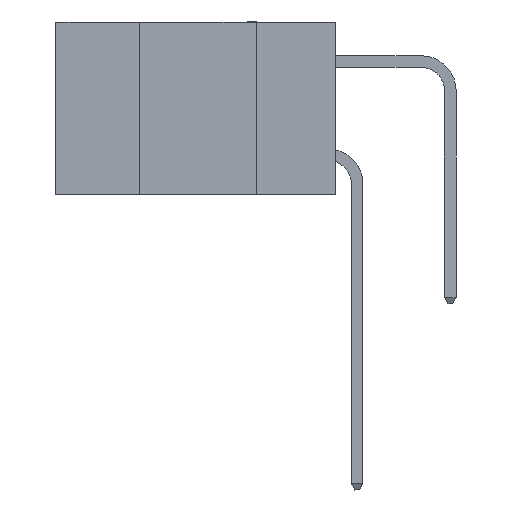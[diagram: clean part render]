
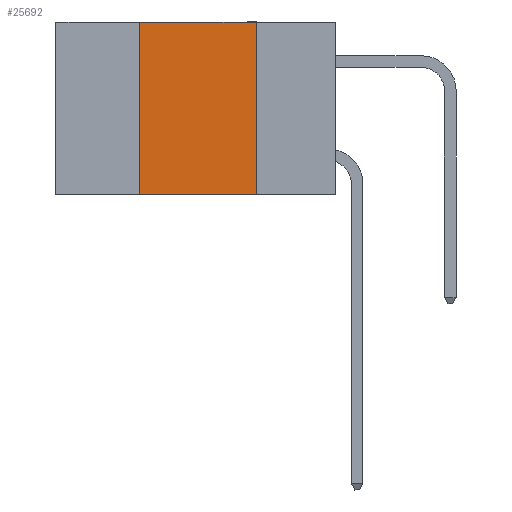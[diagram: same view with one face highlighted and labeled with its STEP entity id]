
A CAD part, left-side view. The second image highlights one B-rep face of the part: STEP entity #25692.
In plain terms, the highlighted planar face has unit normal (-1, 0, 0).
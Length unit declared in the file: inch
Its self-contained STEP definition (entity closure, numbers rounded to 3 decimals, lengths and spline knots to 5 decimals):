
#676 = VERTEX_POINT ( 'NONE', #12379 ) ;
#945 = CARTESIAN_POINT ( 'NONE',  ( 0., 0.17, -0.37 ) ) ;
#1502 = CARTESIAN_POINT ( 'NONE',  ( 0., 0.6, -0.37 ) ) ;
#2795 = ORIENTED_EDGE ( 'NONE', *, *, #4823, .T. ) ;
#4257 = VERTEX_POINT ( 'NONE', #945 ) ;
#4499 = CARTESIAN_POINT ( 'NONE',  ( 0., 0.6, 0. ) ) ;
#4823 = EDGE_CURVE ( 'NONE', #35407, #4257, #29522, .T. ) ;
#5032 = VECTOR ( 'NONE', #8800, 39.37008 ) ;
#7163 = FACE_OUTER_BOUND ( 'NONE', #11681, .T. ) ;
#8735 = ORIENTED_EDGE ( 'NONE', *, *, #37321, .F. ) ;
#8800 = DIRECTION ( 'NONE',  ( 0., 0., 1. ) ) ;
#11099 = VECTOR ( 'NONE', #13797, 39.37008 ) ;
#11681 = EDGE_LOOP ( 'NONE', ( #12983, #15806, #8735, #2795 ) ) ;
#12379 = CARTESIAN_POINT ( 'NONE',  ( 0., 0.17, 0. ) ) ;
#12983 = ORIENTED_EDGE ( 'NONE', *, *, #24397, .F. ) ;
#13346 = VECTOR ( 'NONE', #30147, 39.37008 ) ;
#13797 = DIRECTION ( 'NONE',  ( 0., -1., 0. ) ) ;
#13846 = CARTESIAN_POINT ( 'NONE',  ( 0., 0.17, 0. ) ) ;
#13902 = PLANE ( 'NONE',  #26575 ) ;
#15806 = ORIENTED_EDGE ( 'NONE', *, *, #23138, .F. ) ;
#16578 = DIRECTION ( 'NONE',  ( 0., 0., -1. ) ) ;
#17019 = CARTESIAN_POINT ( 'NONE',  ( 0., 0.42, -0.37 ) ) ;
#17896 = CARTESIAN_POINT ( 'NONE',  ( 0., 0.6, 0. ) ) ;
#19986 = DIRECTION ( 'NONE',  ( 0., 0., -1. ) ) ;
#22091 = CARTESIAN_POINT ( 'NONE',  ( 0., 0.42, 0. ) ) ;
#23138 = EDGE_CURVE ( 'NONE', #24062, #676, #39546, .T. ) ;
#24062 = VERTEX_POINT ( 'NONE', #28172 ) ;
#24397 = EDGE_CURVE ( 'NONE', #676, #4257, #33235, .T. ) ;
#25692 = ADVANCED_FACE ( 'NONE', ( #7163 ), #13902, .F. ) ;
#25836 = VECTOR ( 'NONE', #19986, 39.37008 ) ;
#26575 = AXIS2_PLACEMENT_3D ( 'NONE', #4499, #35155, #16578 ) ;
#28172 = CARTESIAN_POINT ( 'NONE',  ( 0., 0.42, 0. ) ) ;
#29522 = LINE ( 'NONE', #1502, #11099 ) ;
#30147 = DIRECTION ( 'NONE',  ( 0., -1., 0. ) ) ;
#33235 = LINE ( 'NONE', #13846, #25836 ) ;
#35155 = DIRECTION ( 'NONE',  ( 1., 0., 0. ) ) ;
#35407 = VERTEX_POINT ( 'NONE', #17019 ) ;
#36790 = LINE ( 'NONE', #22091, #5032 ) ;
#37321 = EDGE_CURVE ( 'NONE', #35407, #24062, #36790, .T. ) ;
#39546 = LINE ( 'NONE', #17896, #13346 ) ;
